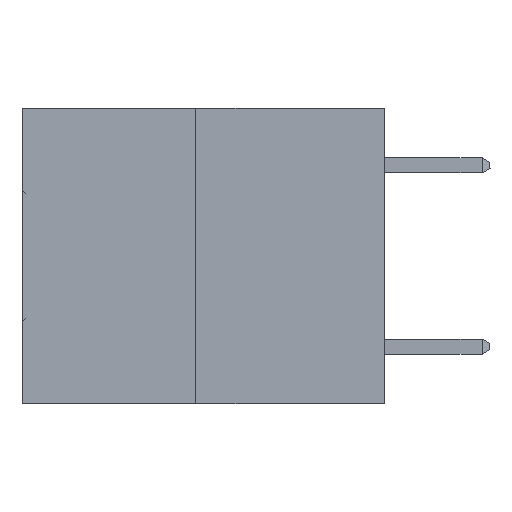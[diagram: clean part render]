
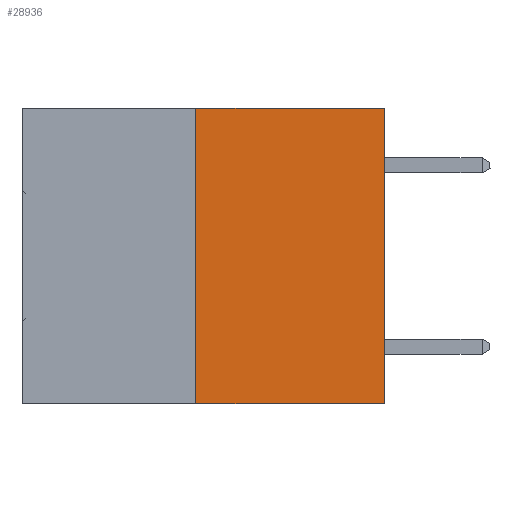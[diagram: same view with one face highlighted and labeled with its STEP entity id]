
A CAD part, left-side view. The second image highlights one B-rep face of the part: STEP entity #28936.
In plain terms, the highlighted planar face has unit normal (-1, 0, 0).
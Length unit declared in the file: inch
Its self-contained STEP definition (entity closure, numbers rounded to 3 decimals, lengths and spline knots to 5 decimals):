
#1918 = DIRECTION ( 'NONE',  ( 0., -1., 0. ) ) ;
#4249 = VERTEX_POINT ( 'NONE', #32091 ) ;
#4273 = DIRECTION ( 'NONE',  ( 0., 0., 1. ) ) ;
#6538 = FACE_OUTER_BOUND ( 'NONE', #11575, .T. ) ;
#7209 = EDGE_CURVE ( 'NONE', #26122, #33578, #23581, .T. ) ;
#7389 = VECTOR ( 'NONE', #1918, 39.37008 ) ;
#7812 = VECTOR ( 'NONE', #10683, 39.37008 ) ;
#7964 = EDGE_CURVE ( 'NONE', #11906, #4249, #31990, .T. ) ;
#8096 = CARTESIAN_POINT ( 'NONE',  ( 0., 0.6, 0. ) ) ;
#9180 = LINE ( 'NONE', #13628, #7389 ) ;
#10683 = DIRECTION ( 'NONE',  ( 0., -1., 0. ) ) ;
#11575 = EDGE_LOOP ( 'NONE', ( #28722, #30581, #19756, #11709 ) ) ;
#11709 = ORIENTED_EDGE ( 'NONE', *, *, #30246, .F. ) ;
#11906 = VERTEX_POINT ( 'NONE', #21847 ) ;
#13628 = CARTESIAN_POINT ( 'NONE',  ( 0., 0.6, -0.49 ) ) ;
#17184 = CARTESIAN_POINT ( 'NONE',  ( 0., 0.312, -0.49 ) ) ;
#18441 = EDGE_CURVE ( 'NONE', #26122, #11906, #9180, .T. ) ;
#19165 = CARTESIAN_POINT ( 'NONE',  ( 0., 0.6, 0. ) ) ;
#19756 = ORIENTED_EDGE ( 'NONE', *, *, #7964, .T. ) ;
#21847 = CARTESIAN_POINT ( 'NONE',  ( 0., 0., -0.49 ) ) ;
#21925 = AXIS2_PLACEMENT_3D ( 'NONE', #8096, #34133, #31481 ) ;
#22464 = CARTESIAN_POINT ( 'NONE',  ( 0., 0.312, -0.49 ) ) ;
#23581 = LINE ( 'NONE', #22464, #26281 ) ;
#26122 = VERTEX_POINT ( 'NONE', #17184 ) ;
#26281 = VECTOR ( 'NONE', #28224, 39.37008 ) ;
#28224 = DIRECTION ( 'NONE',  ( 0., 0., 1. ) ) ;
#28722 = ORIENTED_EDGE ( 'NONE', *, *, #7209, .F. ) ;
#28936 = ADVANCED_FACE ( 'NONE', ( #6538 ), #30469, .F. ) ;
#29789 = VECTOR ( 'NONE', #4273, 39.37008 ) ;
#30246 = EDGE_CURVE ( 'NONE', #33578, #4249, #36420, .T. ) ;
#30469 = PLANE ( 'NONE',  #21925 ) ;
#30581 = ORIENTED_EDGE ( 'NONE', *, *, #18441, .T. ) ;
#30977 = CARTESIAN_POINT ( 'NONE',  ( 0., 0.312, 0. ) ) ;
#31481 = DIRECTION ( 'NONE',  ( 0., 0., -1. ) ) ;
#31990 = LINE ( 'NONE', #32620, #29789 ) ;
#32091 = CARTESIAN_POINT ( 'NONE',  ( 0., 0., 0. ) ) ;
#32620 = CARTESIAN_POINT ( 'NONE',  ( 0., 0., 0. ) ) ;
#33578 = VERTEX_POINT ( 'NONE', #30977 ) ;
#34133 = DIRECTION ( 'NONE',  ( 1., 0., 0. ) ) ;
#36420 = LINE ( 'NONE', #19165, #7812 ) ;
